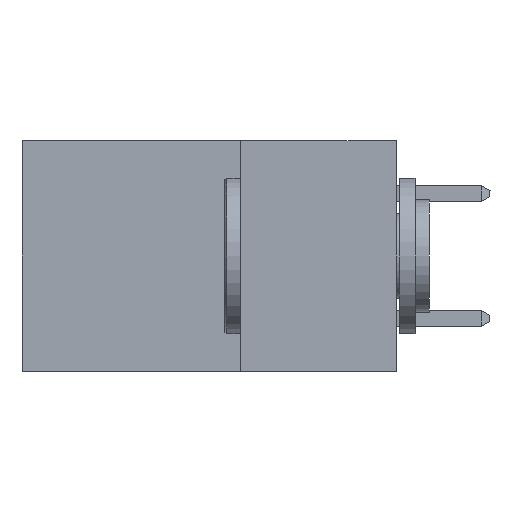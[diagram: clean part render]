
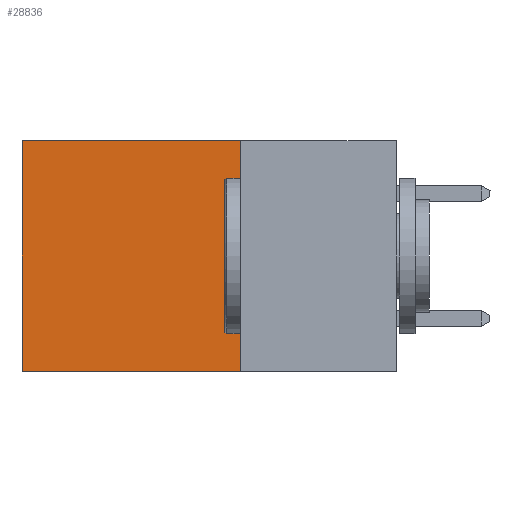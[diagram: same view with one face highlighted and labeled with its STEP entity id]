
A CAD part, left-side view. The second image highlights one B-rep face of the part: STEP entity #28836.
In plain terms, the highlighted planar face has unit normal (-1, 0, 0).
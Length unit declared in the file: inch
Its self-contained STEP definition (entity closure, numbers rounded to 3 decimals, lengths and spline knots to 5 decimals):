
#2544 = LINE ( 'NONE', #7515, #19857 ) ;
#2910 = FACE_OUTER_BOUND ( 'NONE', #25428, .T. ) ;
#3267 = CARTESIAN_POINT ( 'NONE',  ( 0.298, 0.25, 0. ) ) ;
#3301 = DIRECTION ( 'NONE',  ( 0., 1., 0. ) ) ;
#3391 = EDGE_CURVE ( 'NONE', #15070, #5389, #4823, .T. ) ;
#4823 = LINE ( 'NONE', #8493, #31061 ) ;
#5301 = CARTESIAN_POINT ( 'NONE',  ( 0.298, 0.6, -0.37 ) ) ;
#5389 = VERTEX_POINT ( 'NONE', #24532 ) ;
#7103 = PLANE ( 'NONE',  #18442 ) ;
#7515 = CARTESIAN_POINT ( 'NONE',  ( 0.298, 0.25, -0.37 ) ) ;
#8303 = ORIENTED_EDGE ( 'NONE', *, *, #30359, .T. ) ;
#8349 = DIRECTION ( 'NONE',  ( 0., 0., -1. ) ) ;
#8493 = CARTESIAN_POINT ( 'NONE',  ( 0.298, 0.25, 0. ) ) ;
#8556 = LINE ( 'NONE', #20142, #21688 ) ;
#8675 = ORIENTED_EDGE ( 'NONE', *, *, #3391, .T. ) ;
#9482 = VERTEX_POINT ( 'NONE', #11116 ) ;
#9837 = CARTESIAN_POINT ( 'NONE',  ( 0.298, 0.25, 0. ) ) ;
#10118 = EDGE_CURVE ( 'NONE', #15070, #9482, #18471, .T. ) ;
#10625 = DIRECTION ( 'NONE',  ( 1., 0., 0. ) ) ;
#11116 = CARTESIAN_POINT ( 'NONE',  ( 0.298, 0.25, -0.37 ) ) ;
#13222 = ORIENTED_EDGE ( 'NONE', *, *, #28278, .F. ) ;
#14932 = DIRECTION ( 'NONE',  ( 0., 0., -1. ) ) ;
#15070 = VERTEX_POINT ( 'NONE', #9837 ) ;
#16669 = DIRECTION ( 'NONE',  ( 0., 0., -1. ) ) ;
#18442 = AXIS2_PLACEMENT_3D ( 'NONE', #20329, #10625, #16669 ) ;
#18471 = LINE ( 'NONE', #3267, #23391 ) ;
#19857 = VECTOR ( 'NONE', #28574, 39.37008 ) ;
#20142 = CARTESIAN_POINT ( 'NONE',  ( 0.298, 0.6, 0. ) ) ;
#20329 = CARTESIAN_POINT ( 'NONE',  ( 0.298, 0.25, 0. ) ) ;
#21688 = VECTOR ( 'NONE', #14932, 39.37008 ) ;
#23391 = VECTOR ( 'NONE', #8349, 39.37008 ) ;
#24532 = CARTESIAN_POINT ( 'NONE',  ( 0.298, 0.6, 0. ) ) ;
#25428 = EDGE_LOOP ( 'NONE', ( #8303, #13222, #31084, #8675 ) ) ;
#28259 = VERTEX_POINT ( 'NONE', #5301 ) ;
#28278 = EDGE_CURVE ( 'NONE', #9482, #28259, #2544, .T. ) ;
#28574 = DIRECTION ( 'NONE',  ( 0., 1., 0. ) ) ;
#28836 = ADVANCED_FACE ( 'NONE', ( #2910 ), #7103, .F. ) ;
#30359 = EDGE_CURVE ( 'NONE', #5389, #28259, #8556, .T. ) ;
#31061 = VECTOR ( 'NONE', #3301, 39.37008 ) ;
#31084 = ORIENTED_EDGE ( 'NONE', *, *, #10118, .F. ) ;
